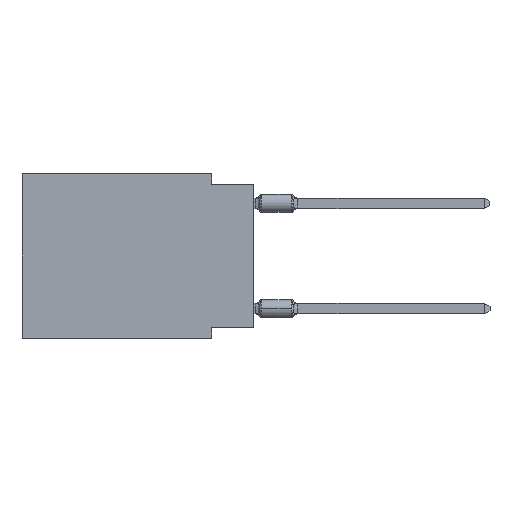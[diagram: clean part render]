
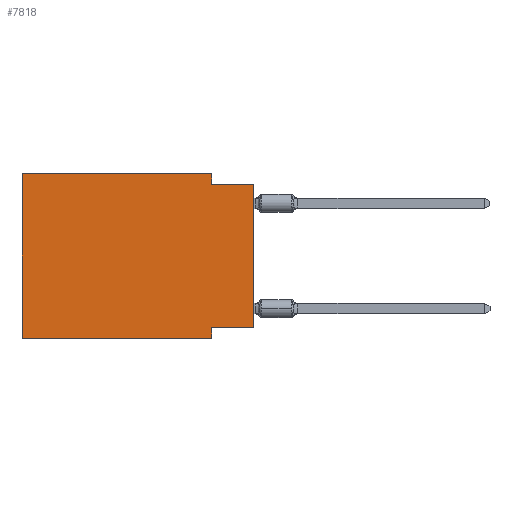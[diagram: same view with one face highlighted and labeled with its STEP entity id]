
A CAD part, left-side view. The second image highlights one B-rep face of the part: STEP entity #7818.
In plain terms, the highlighted planar face has unit normal (-1, 0, 0).
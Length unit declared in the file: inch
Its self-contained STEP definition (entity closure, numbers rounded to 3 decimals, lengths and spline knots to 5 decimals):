
#111 = DIRECTION ( 'NONE',  ( 0., 0., 1. ) ) ;
#479 = LINE ( 'NONE', #17440, #2216 ) ;
#565 = ORIENTED_EDGE ( 'NONE', *, *, #3784, .F. ) ;
#785 = LINE ( 'NONE', #16624, #6290 ) ;
#842 = LINE ( 'NONE', #16298, #13012 ) ;
#1038 = DIRECTION ( 'NONE',  ( 0., 0., -1. ) ) ;
#1269 = CARTESIAN_POINT ( 'NONE',  ( 0., 0.1, 0. ) ) ;
#2020 = ORIENTED_EDGE ( 'NONE', *, *, #18392, .T. ) ;
#2216 = VECTOR ( 'NONE', #6740, 39.37008 ) ;
#2363 = VERTEX_POINT ( 'NONE', #17817 ) ;
#3644 = DIRECTION ( 'NONE',  ( 0., 0., 1. ) ) ;
#3690 = EDGE_CURVE ( 'NONE', #9639, #6444, #14526, .T. ) ;
#3784 = EDGE_CURVE ( 'NONE', #18205, #2363, #785, .T. ) ;
#3821 = EDGE_LOOP ( 'NONE', ( #9179, #9691, #8467, #5507, #9983, #2020, #15339, #565 ) ) ;
#3904 = DIRECTION ( 'NONE',  ( 0., -1., 0. ) ) ;
#4095 = LINE ( 'NONE', #12144, #4414 ) ;
#4232 = VERTEX_POINT ( 'NONE', #4576 ) ;
#4271 = EDGE_CURVE ( 'NONE', #18205, #4232, #12634, .T. ) ;
#4328 = VERTEX_POINT ( 'NONE', #15468 ) ;
#4414 = VECTOR ( 'NONE', #1038, 39.37008 ) ;
#4576 = CARTESIAN_POINT ( 'NONE',  ( 0., 0., -0.025 ) ) ;
#5002 = CARTESIAN_POINT ( 'NONE',  ( 0., 0.55, 0. ) ) ;
#5507 = ORIENTED_EDGE ( 'NONE', *, *, #10327, .F. ) ;
#5557 = EDGE_CURVE ( 'NONE', #16137, #8375, #15670, .T. ) ;
#6082 = PLANE ( 'NONE',  #18433 ) ;
#6290 = VECTOR ( 'NONE', #19358, 39.37008 ) ;
#6350 = LINE ( 'NONE', #9496, #18738 ) ;
#6444 = VERTEX_POINT ( 'NONE', #5002 ) ;
#6740 = DIRECTION ( 'NONE',  ( 0., -1., 0. ) ) ;
#7119 = EDGE_CURVE ( 'NONE', #8375, #4232, #6350, .T. ) ;
#7587 = DIRECTION ( 'NONE',  ( 0., 0., -1. ) ) ;
#7818 = ADVANCED_FACE ( 'NONE', ( #12237 ), #6082, .F. ) ;
#8375 = VERTEX_POINT ( 'NONE', #11205 ) ;
#8467 = ORIENTED_EDGE ( 'NONE', *, *, #5557, .F. ) ;
#9179 = ORIENTED_EDGE ( 'NONE', *, *, #4271, .T. ) ;
#9496 = CARTESIAN_POINT ( 'NONE',  ( 0., 0., -0.025 ) ) ;
#9639 = VERTEX_POINT ( 'NONE', #18450 ) ;
#9691 = ORIENTED_EDGE ( 'NONE', *, *, #7119, .F. ) ;
#9983 = ORIENTED_EDGE ( 'NONE', *, *, #3690, .F. ) ;
#10311 = VECTOR ( 'NONE', #111, 39.37008 ) ;
#10327 = EDGE_CURVE ( 'NONE', #6444, #16137, #842, .T. ) ;
#11205 = CARTESIAN_POINT ( 'NONE',  ( 0., 0.1, -0.025 ) ) ;
#11258 = VECTOR ( 'NONE', #14041, 39.37008 ) ;
#12144 = CARTESIAN_POINT ( 'NONE',  ( 0., 0.1, -0.39 ) ) ;
#12237 = FACE_OUTER_BOUND ( 'NONE', #3821, .T. ) ;
#12498 = CARTESIAN_POINT ( 'NONE',  ( 0., 0., -0.365 ) ) ;
#12634 = LINE ( 'NONE', #18589, #10311 ) ;
#13012 = VECTOR ( 'NONE', #3904, 39.37008 ) ;
#14041 = DIRECTION ( 'NONE',  ( 0., 0., -1. ) ) ;
#14346 = CARTESIAN_POINT ( 'NONE',  ( 0., 0.1, 0. ) ) ;
#14526 = LINE ( 'NONE', #17448, #17570 ) ;
#14825 = EDGE_CURVE ( 'NONE', #2363, #4328, #4095, .T. ) ;
#15339 = ORIENTED_EDGE ( 'NONE', *, *, #14825, .F. ) ;
#15468 = CARTESIAN_POINT ( 'NONE',  ( 0., 0.1, -0.39 ) ) ;
#15670 = LINE ( 'NONE', #14346, #11258 ) ;
#16137 = VERTEX_POINT ( 'NONE', #1269 ) ;
#16298 = CARTESIAN_POINT ( 'NONE',  ( 0., 0.55, 0. ) ) ;
#16624 = CARTESIAN_POINT ( 'NONE',  ( 0., 0., -0.365 ) ) ;
#16783 = DIRECTION ( 'NONE',  ( 1., 0., 0. ) ) ;
#17440 = CARTESIAN_POINT ( 'NONE',  ( 0., 0.55, -0.39 ) ) ;
#17448 = CARTESIAN_POINT ( 'NONE',  ( 0., 0.55, 0. ) ) ;
#17457 = DIRECTION ( 'NONE',  ( 0., -1., 0. ) ) ;
#17570 = VECTOR ( 'NONE', #3644, 39.37008 ) ;
#17817 = CARTESIAN_POINT ( 'NONE',  ( 0., 0.1, -0.365 ) ) ;
#18205 = VERTEX_POINT ( 'NONE', #12498 ) ;
#18392 = EDGE_CURVE ( 'NONE', #9639, #4328, #479, .T. ) ;
#18433 = AXIS2_PLACEMENT_3D ( 'NONE', #18500, #16783, #7587 ) ;
#18450 = CARTESIAN_POINT ( 'NONE',  ( 0., 0.55, -0.39 ) ) ;
#18500 = CARTESIAN_POINT ( 'NONE',  ( 0., 0.55, 0. ) ) ;
#18589 = CARTESIAN_POINT ( 'NONE',  ( 0., 0., 0. ) ) ;
#18738 = VECTOR ( 'NONE', #17457, 39.37008 ) ;
#19358 = DIRECTION ( 'NONE',  ( 0., 1., 0. ) ) ;
